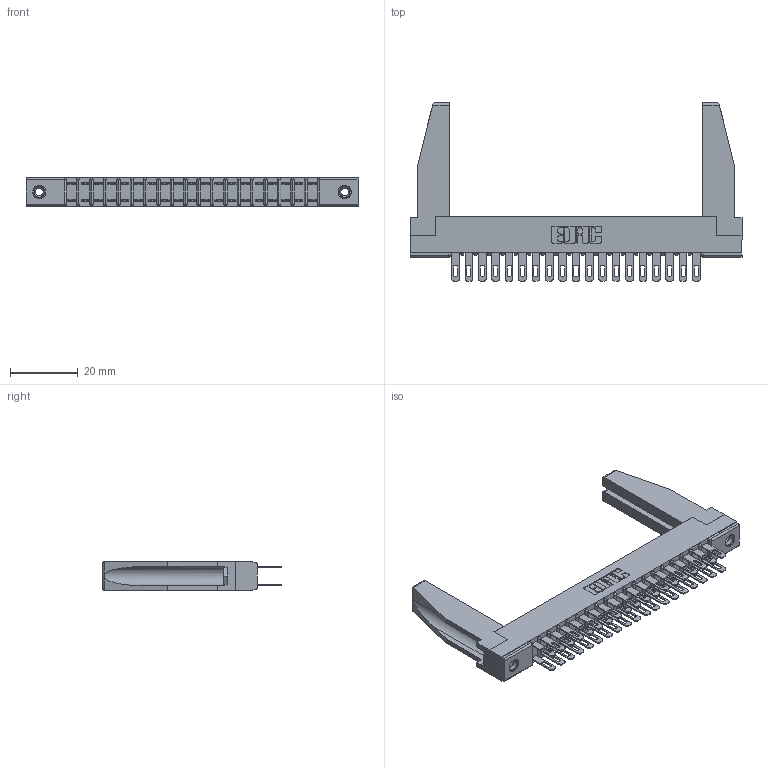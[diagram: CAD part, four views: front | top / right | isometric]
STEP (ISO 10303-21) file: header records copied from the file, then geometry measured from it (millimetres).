
FILE_DESCRIPTION (( 'STEP AP203' ), '1' );
FILE_NAME ('307-038-400-278.STEP', '2020-09-29T18:23:41', ( '' ), ( '' ), 'SwSTEP 2.0', 'SolidWorks 2020', '' );
FILE_SCHEMA (( 'CONFIG_CONTROL_DESIGN' ));
Length unit declared in the file: inch
Products named in the file (5): 307-220-078; 345-250-001_345-250-001-102; 307 Part_.156 Dia Mounting Holes; 307-038-400-278; 307-290-001_500
Assembly tree (43 placements, depth 2):
  307-038-400-278
    307 Part_.156 Dia Mounting Holes
    307-290-001_500  x38
    307-220-078  x2
    345-250-001_345-250-001-102  x2
Bounding box: 98.3 x 52.88 x 8.71 mm (x, y, z)
Volume: 10532.3 mm3; surface area: 15821 mm2
Topology: 43 solids, 43 shells, 2016 faces, 5593 edges, 3614 vertices
Faces by surface type: plane 1294, cylinder 666, sphere 40, cone 12, torus 4
Entity records: 22145 total; most frequent: CARTESIAN_POINT 3637, ORIENTED_EDGE 3560, DIRECTION 3528, EDGE_CURVE 1780, LINE 1358, VECTOR 1358, VERTEX_POINT 1152, AXIS2_PLACEMENT_3D 1085
